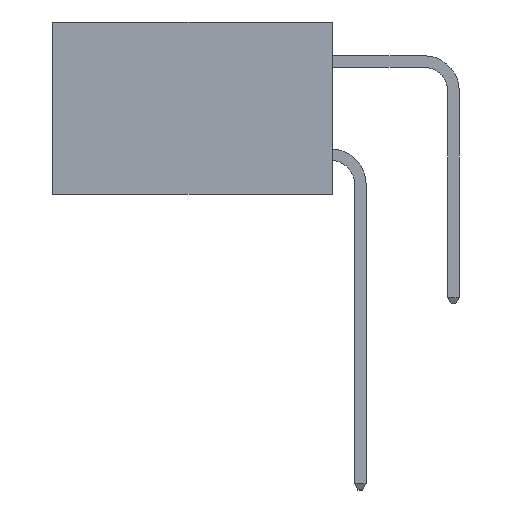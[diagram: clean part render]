
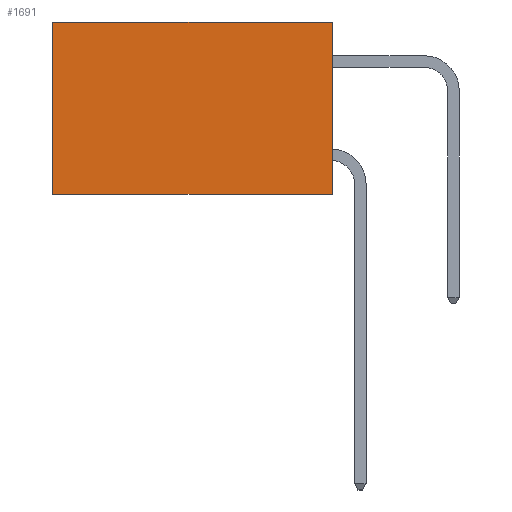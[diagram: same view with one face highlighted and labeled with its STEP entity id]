
A CAD part, left-side view. The second image highlights one B-rep face of the part: STEP entity #1691.
In plain terms, the highlighted planar face has unit normal (-1, 0, 0).
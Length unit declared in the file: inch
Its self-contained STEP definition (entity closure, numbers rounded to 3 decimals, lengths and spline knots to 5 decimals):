
#75 = EDGE_LOOP ( 'NONE', ( #9245, #7854, #5607, #3155 ) ) ;
#462 = EDGE_CURVE ( 'NONE', #13239, #4544, #4451, .T. ) ;
#1172 = CARTESIAN_POINT ( 'NONE',  ( 0.2615, 0., 0. ) ) ;
#1508 = LINE ( 'NONE', #5324, #12193 ) ;
#1691 = ADVANCED_FACE ( 'NONE', ( #6761 ), #9656, .F. ) ;
#1757 = DIRECTION ( 'NONE',  ( 0., 0., -1. ) ) ;
#1849 = DIRECTION ( 'NONE',  ( 0., 1., 0. ) ) ;
#2085 = EDGE_CURVE ( 'NONE', #6552, #4544, #1508, .T. ) ;
#2817 = AXIS2_PLACEMENT_3D ( 'NONE', #9647, #9621, #9615 ) ;
#3155 = ORIENTED_EDGE ( 'NONE', *, *, #6973, .T. ) ;
#3517 = VECTOR ( 'NONE', #1849, 39.37008 ) ;
#4451 = LINE ( 'NONE', #10550, #7125 ) ;
#4544 = VERTEX_POINT ( 'NONE', #11006 ) ;
#5324 = CARTESIAN_POINT ( 'NONE',  ( 0.2615, 0., -0.37 ) ) ;
#5342 = DIRECTION ( 'NONE',  ( 0., 1., 0. ) ) ;
#5417 = EDGE_CURVE ( 'NONE', #13048, #6552, #12771, .T. ) ;
#5607 = ORIENTED_EDGE ( 'NONE', *, *, #5417, .F. ) ;
#6552 = VERTEX_POINT ( 'NONE', #9252 ) ;
#6761 = FACE_OUTER_BOUND ( 'NONE', #75, .T. ) ;
#6973 = EDGE_CURVE ( 'NONE', #13048, #13239, #9124, .T. ) ;
#6985 = CARTESIAN_POINT ( 'NONE',  ( 0.2615, 0.6, 0. ) ) ;
#7125 = VECTOR ( 'NONE', #1757, 39.37008 ) ;
#7211 = VECTOR ( 'NONE', #9690, 39.37008 ) ;
#7854 = ORIENTED_EDGE ( 'NONE', *, *, #2085, .F. ) ;
#9124 = LINE ( 'NONE', #1172, #3517 ) ;
#9245 = ORIENTED_EDGE ( 'NONE', *, *, #462, .T. ) ;
#9252 = CARTESIAN_POINT ( 'NONE',  ( 0.2615, 0., -0.37 ) ) ;
#9615 = DIRECTION ( 'NONE',  ( 0., 0., -1. ) ) ;
#9621 = DIRECTION ( 'NONE',  ( 1., 0., 0. ) ) ;
#9647 = CARTESIAN_POINT ( 'NONE',  ( 0.2615, 0., -0.37 ) ) ;
#9656 = PLANE ( 'NONE',  #2817 ) ;
#9690 = DIRECTION ( 'NONE',  ( 0., 0., -1. ) ) ;
#10550 = CARTESIAN_POINT ( 'NONE',  ( 0.2615, 0.6, -0.37 ) ) ;
#10932 = CARTESIAN_POINT ( 'NONE',  ( 0.2615, 0., 0. ) ) ;
#11006 = CARTESIAN_POINT ( 'NONE',  ( 0.2615, 0.6, -0.37 ) ) ;
#11543 = CARTESIAN_POINT ( 'NONE',  ( 0.2615, 0., -0.37 ) ) ;
#12193 = VECTOR ( 'NONE', #5342, 39.37008 ) ;
#12771 = LINE ( 'NONE', #11543, #7211 ) ;
#13048 = VERTEX_POINT ( 'NONE', #10932 ) ;
#13239 = VERTEX_POINT ( 'NONE', #6985 ) ;
